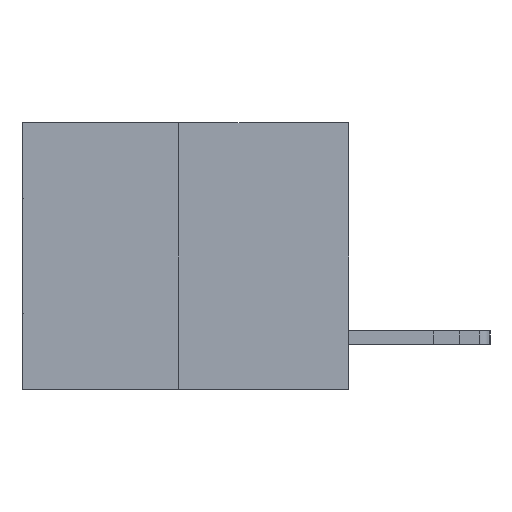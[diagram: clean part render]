
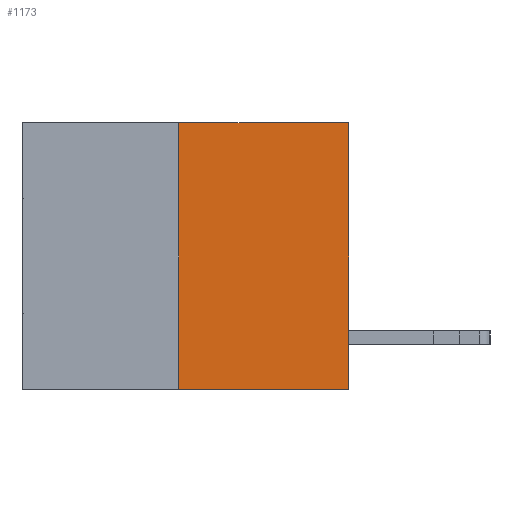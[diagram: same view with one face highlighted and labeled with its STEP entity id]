
A CAD part, left-side view. The second image highlights one B-rep face of the part: STEP entity #1173.
In plain terms, the highlighted planar face has unit normal (-1, 0, 0).
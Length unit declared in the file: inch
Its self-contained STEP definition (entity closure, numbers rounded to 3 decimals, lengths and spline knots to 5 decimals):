
#307 = VERTEX_POINT ( 'NONE', #29869 ) ;
#600 = LINE ( 'NONE', #13299, #23164 ) ;
#1173 = ADVANCED_FACE ( 'NONE', ( #19307 ), #11392, .F. ) ;
#1416 = VERTEX_POINT ( 'NONE', #16808 ) ;
#1445 = LINE ( 'NONE', #4954, #23268 ) ;
#2413 = LINE ( 'NONE', #20641, #10342 ) ;
#2833 = DIRECTION ( 'NONE',  ( 0., 0., 1. ) ) ;
#3518 = EDGE_CURVE ( 'NONE', #1416, #7177, #1445, .T. ) ;
#3854 = CARTESIAN_POINT ( 'NONE',  ( 0., 0.6, 0. ) ) ;
#4954 = CARTESIAN_POINT ( 'NONE',  ( 0., 0., 0. ) ) ;
#6049 = DIRECTION ( 'NONE',  ( 0., 0., 1. ) ) ;
#6145 = AXIS2_PLACEMENT_3D ( 'NONE', #3854, #11484, #13417 ) ;
#6475 = LINE ( 'NONE', #28709, #26775 ) ;
#7177 = VERTEX_POINT ( 'NONE', #19456 ) ;
#8653 = EDGE_CURVE ( 'NONE', #307, #30573, #600, .T. ) ;
#8731 = EDGE_CURVE ( 'NONE', #307, #1416, #2413, .T. ) ;
#10342 = VECTOR ( 'NONE', #27365, 39.37008 ) ;
#11392 = PLANE ( 'NONE',  #6145 ) ;
#11484 = DIRECTION ( 'NONE',  ( 1., 0., 0. ) ) ;
#13299 = CARTESIAN_POINT ( 'NONE',  ( 0., 0.312, -0.49 ) ) ;
#13417 = DIRECTION ( 'NONE',  ( 0., 0., -1. ) ) ;
#16808 = CARTESIAN_POINT ( 'NONE',  ( 0., 0., -0.49 ) ) ;
#16892 = ORIENTED_EDGE ( 'NONE', *, *, #3518, .T. ) ;
#17185 = ORIENTED_EDGE ( 'NONE', *, *, #8653, .F. ) ;
#19307 = FACE_OUTER_BOUND ( 'NONE', #30634, .T. ) ;
#19440 = ORIENTED_EDGE ( 'NONE', *, *, #8731, .T. ) ;
#19456 = CARTESIAN_POINT ( 'NONE',  ( 0., 0., 0. ) ) ;
#20641 = CARTESIAN_POINT ( 'NONE',  ( 0., 0.6, -0.49 ) ) ;
#23164 = VECTOR ( 'NONE', #6049, 39.37008 ) ;
#23268 = VECTOR ( 'NONE', #2833, 39.37008 ) ;
#23965 = DIRECTION ( 'NONE',  ( 0., -1., 0. ) ) ;
#26469 = CARTESIAN_POINT ( 'NONE',  ( 0., 0.312, 0. ) ) ;
#26692 = EDGE_CURVE ( 'NONE', #30573, #7177, #6475, .T. ) ;
#26775 = VECTOR ( 'NONE', #23965, 39.37008 ) ;
#27365 = DIRECTION ( 'NONE',  ( 0., -1., 0. ) ) ;
#28709 = CARTESIAN_POINT ( 'NONE',  ( 0., 0.6, 0. ) ) ;
#28823 = ORIENTED_EDGE ( 'NONE', *, *, #26692, .F. ) ;
#29869 = CARTESIAN_POINT ( 'NONE',  ( 0., 0.312, -0.49 ) ) ;
#30573 = VERTEX_POINT ( 'NONE', #26469 ) ;
#30634 = EDGE_LOOP ( 'NONE', ( #17185, #19440, #16892, #28823 ) ) ;
